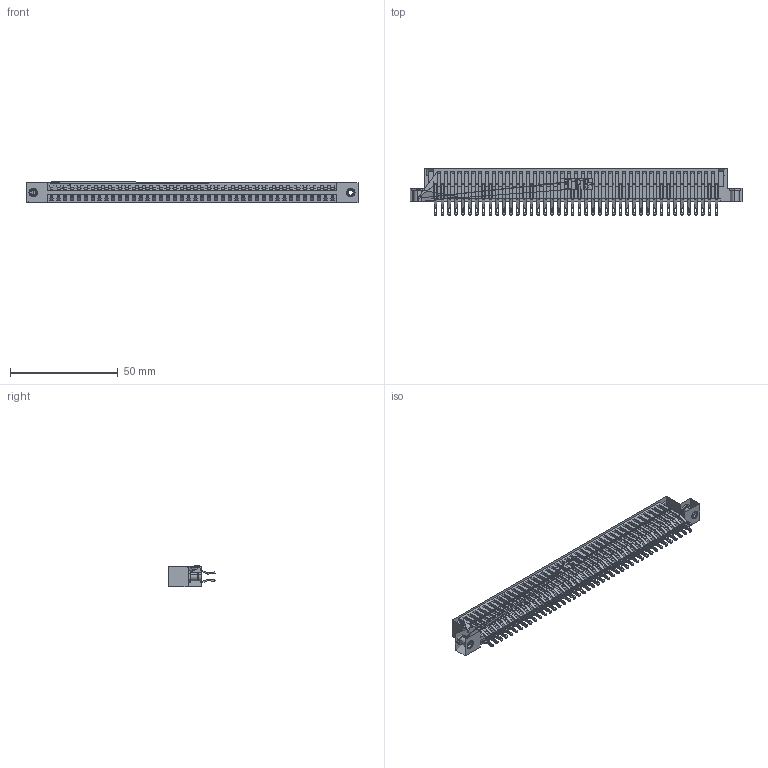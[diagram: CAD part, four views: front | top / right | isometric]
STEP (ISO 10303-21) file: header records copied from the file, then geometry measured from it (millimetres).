
FILE_DESCRIPTION (( 'STEP AP203' ), '1' );
FILE_NAME ('346-084-555-208.STEP', '2022-05-25T20:27:38', ( '' ), ( '' ), 'SwSTEP 2.0', 'SolidWorks 2020', '' );
FILE_SCHEMA (( 'CONFIG_CONTROL_DESIGN' ));
Length unit declared in the file: inch
Products named in the file (4): 345-292-001_555 Tail; 346 Part_Flush Mounting Lugs - 0.156 Dia-TI; 346-084-555-208; 345-250-001_345-250-003-102
Assembly tree (87 placements, depth 2):
  346-084-555-208
    346 Part_Flush Mounting Lugs - 0.156 Dia-TI
    345-292-001_555 Tail  x84
    345-250-001_345-250-003-102  x2
Bounding box: 153.92 x 21.46 x 10.03 mm (x, y, z)
Volume: 14666 mm3; surface area: 21382.3 mm2
Topology: 87 solids, 87 shells, 5054 faces, 15837 edges, 10567 vertices
Faces by surface type: plane 2880, cylinder 2158, cone 12, torus 4
Entity records: 28922 total; most frequent: CARTESIAN_POINT 4785, ORIENTED_EDGE 4682, DIRECTION 4263, EDGE_CURVE 2341, VECTOR 2001, LINE 2001, VERTEX_POINT 1556, AXIS2_PLACEMENT_3D 1131
